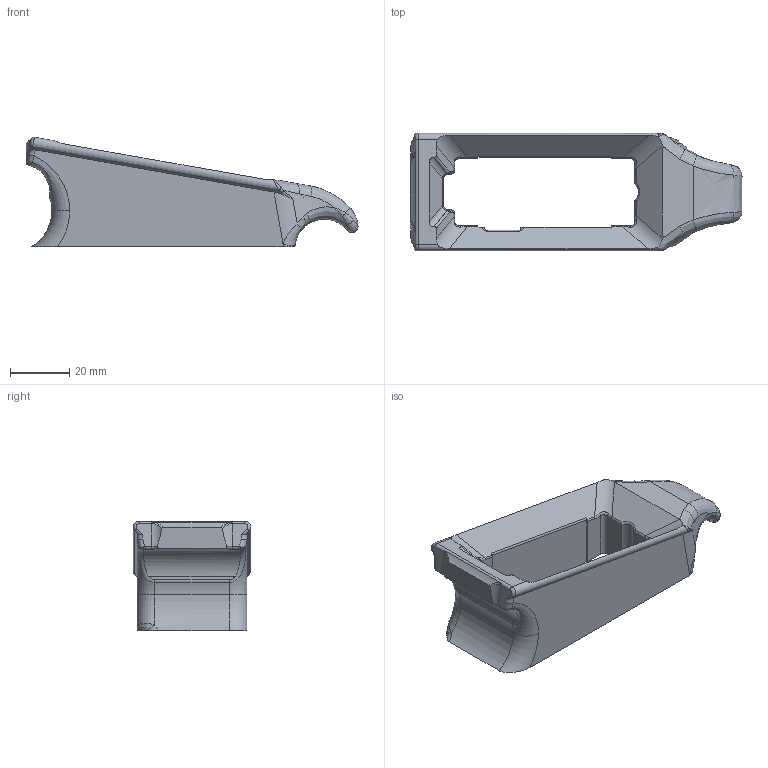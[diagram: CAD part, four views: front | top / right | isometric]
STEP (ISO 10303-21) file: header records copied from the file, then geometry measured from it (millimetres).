
FILE_DESCRIPTION (( 'STEP AP214' ), '1' );
FILE_NAME ('Magwell_3b.STEP', '2013-09-01T16:46:28', ( 'Asher' ), ( '' ), 'SwSTEP 2.0', 'SolidWorks 2013', '' );
FILE_SCHEMA (( 'AUTOMOTIVE_DESIGN' ));
Length unit declared in the file: millimetre
Products named in the file (1): Magwell_3b
Bounding box: 112.19 x 39.78 x 37.04 mm (x, y, z)
Volume: 46993.1 mm3; surface area: 16257.1 mm2
Topology: 1 solids, 1 shells, 201 faces, 528 edges, 321 vertices
Faces by surface type: bspline 81, cylinder 55, plane 51, torus 12, sphere 2
Entity records: 9942 total; most frequent: CARTESIAN_POINT 5480, ORIENTED_EDGE 1042, DIRECTION 651, EDGE_CURVE 521, VERTEX_POINT 321, AXIS2_PLACEMENT_3D 235, EDGE_LOOP 202, FACE_OUTER_BOUND 201
